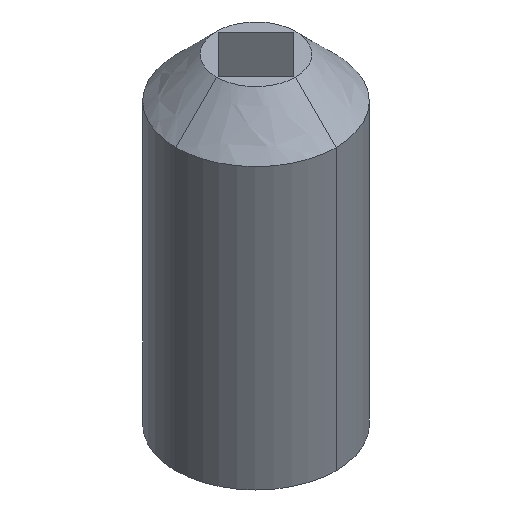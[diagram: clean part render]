
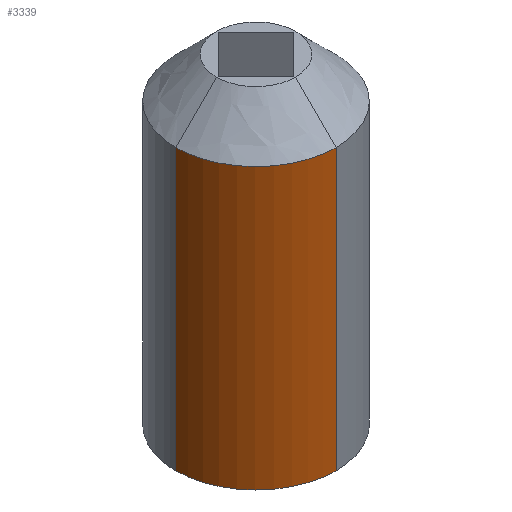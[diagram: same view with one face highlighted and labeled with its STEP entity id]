
A CAD part, isometric view. The second image highlights one B-rep face of the part: STEP entity #3339.
In plain terms, the highlighted free-form (B-spline) face has degree [2, 1] with [3, 2] control points.
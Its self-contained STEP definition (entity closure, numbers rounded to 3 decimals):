
#150 = VERTEX_POINT('',#151);
#151 = CARTESIAN_POINT('',(0.,-9.525,33.274));
#164 = ( BOUNDED_SURFACE() B_SPLINE_SURFACE(2,1,(
    (#165,#166)
    ,(#167,#168)
,(#169,#170
    )),.UNSPECIFIED.,.F.,.F.,.F.) B_SPLINE_SURFACE_WITH_KNOTS((3,3),(2,2
    ),(0.,1.),(0.,1.),.PIECEWISE_BEZIER_KNOTS.) 
GEOMETRIC_REPRESENTATION_ITEM() RATIONAL_B_SPLINE_SURFACE((
    (1.,1.)
    ,(0.707,0.707)
,(1.,1.))) REPRESENTATION_ITEM('') SURFACE() );
#165 = CARTESIAN_POINT('',(-4.699,0.,38.1));
#166 = CARTESIAN_POINT('',(-9.525,0.,33.274));
#167 = CARTESIAN_POINT('',(-4.699,-4.699,38.1));
#168 = CARTESIAN_POINT('',(-9.525,-9.525,33.274));
#169 = CARTESIAN_POINT('',(0.,-4.699,38.1));
#170 = CARTESIAN_POINT('',(0.,-9.525,33.274));
#214 = ( BOUNDED_SURFACE() B_SPLINE_SURFACE(2,1,(
    (#215,#216)
    ,(#217,#218)
,(#219,#220
    )),.UNSPECIFIED.,.F.,.F.,.F.) B_SPLINE_SURFACE_WITH_KNOTS((3,3),(2,2
    ),(0.,1.),(0.,1.),.PIECEWISE_BEZIER_KNOTS.) 
GEOMETRIC_REPRESENTATION_ITEM() RATIONAL_B_SPLINE_SURFACE((
    (1.,1.)
    ,(0.707,0.707)
,(1.,1.))) REPRESENTATION_ITEM('') SURFACE() );
#215 = CARTESIAN_POINT('',(0.,-9.525,33.274));
#216 = CARTESIAN_POINT('',(0.,-9.525,0.));
#217 = CARTESIAN_POINT('',(9.525,-9.525,33.274));
#218 = CARTESIAN_POINT('',(9.525,-9.525,0.));
#219 = CARTESIAN_POINT('',(9.525,0.,33.274));
#220 = CARTESIAN_POINT('',(9.525,0.,0.));
#1573 = VERTEX_POINT('',#1574);
#1574 = CARTESIAN_POINT('',(-9.525,0.,33.274));
#1608 = ( BOUNDED_SURFACE() B_SPLINE_SURFACE(2,1,(
    (#1609,#1610)
    ,(#1611,#1612)
    ,(#1613,#1614
)),.UNSPECIFIED.,.F.,.F.,.F.) B_SPLINE_SURFACE_WITH_KNOTS((3,3),(2,2),(
    0.,1.),(0.,1.),.PIECEWISE_BEZIER_KNOTS.) 
GEOMETRIC_REPRESENTATION_ITEM() RATIONAL_B_SPLINE_SURFACE((
    (1.,1.)
    ,(0.707,0.707)
,(1.,1.))) REPRESENTATION_ITEM('') SURFACE() );
#1609 = CARTESIAN_POINT('',(0.,9.525,33.274));
#1610 = CARTESIAN_POINT('',(0.,9.525,0.));
#1611 = CARTESIAN_POINT('',(-9.525,9.525,33.274));
#1612 = CARTESIAN_POINT('',(-9.525,9.525,0.));
#1613 = CARTESIAN_POINT('',(-9.525,0.,33.274));
#1614 = CARTESIAN_POINT('',(-9.525,0.,0.));
#1684 = PLANE('',#1685);
#1685 = AXIS2_PLACEMENT_3D('',#1686,#1687,#1688);
#1686 = CARTESIAN_POINT('',(9.525,0.,0.));
#1687 = DIRECTION('',(0.,0.,-1.));
#1688 = DIRECTION('',(-1.,0.,0.));
#1702 = EDGE_CURVE('',#1573,#150,#1703,.T.);
#1703 = SURFACE_CURVE('',#1704,(#1708,#1715),.PCURVE_S1.);
#1704 = ( BOUNDED_CURVE() B_SPLINE_CURVE(2,(#1705,#1706,#1707),
.UNSPECIFIED.,.F.,.F.) B_SPLINE_CURVE_WITH_KNOTS((3,3),(0.,1.),
.PIECEWISE_BEZIER_KNOTS.) CURVE() GEOMETRIC_REPRESENTATION_ITEM() 
RATIONAL_B_SPLINE_CURVE((1.,0.707,1.)) REPRESENTATION_ITEM('') 
  );
#1705 = CARTESIAN_POINT('',(-9.525,0.,33.274));
#1706 = CARTESIAN_POINT('',(-9.525,-9.525,33.274));
#1707 = CARTESIAN_POINT('',(0.,-9.525,33.274));
#1708 = PCURVE('',#164,#1709);
#1709 = DEFINITIONAL_REPRESENTATION('',(#1710),#1714);
#1710 = LINE('',#1711,#1712);
#1711 = CARTESIAN_POINT('',(0.,1.));
#1712 = VECTOR('',#1713,1.);
#1713 = DIRECTION('',(1.,0.));
#1714 = ( GEOMETRIC_REPRESENTATION_CONTEXT(2) 
PARAMETRIC_REPRESENTATION_CONTEXT() REPRESENTATION_CONTEXT('2D SPACE',''
  ) );
#1715 = PCURVE('',#1716,#1723);
#1716 = ( BOUNDED_SURFACE() B_SPLINE_SURFACE(2,1,(
    (#1717,#1718)
    ,(#1719,#1720)
    ,(#1721,#1722
)),.UNSPECIFIED.,.F.,.F.,.F.) B_SPLINE_SURFACE_WITH_KNOTS((3,3),(2,2),(
    0.,1.),(0.,1.),.PIECEWISE_BEZIER_KNOTS.) 
GEOMETRIC_REPRESENTATION_ITEM() RATIONAL_B_SPLINE_SURFACE((
    (1.,1.)
    ,(0.707,0.707)
,(1.,1.))) REPRESENTATION_ITEM('') SURFACE() );
#1717 = CARTESIAN_POINT('',(-9.525,0.,33.274));
#1718 = CARTESIAN_POINT('',(-9.525,0.,0.));
#1719 = CARTESIAN_POINT('',(-9.525,-9.525,33.274));
#1720 = CARTESIAN_POINT('',(-9.525,-9.525,0.));
#1721 = CARTESIAN_POINT('',(0.,-9.525,33.274));
#1722 = CARTESIAN_POINT('',(0.,-9.525,0.));
#1723 = DEFINITIONAL_REPRESENTATION('',(#1724),#1728);
#1724 = LINE('',#1725,#1726);
#1725 = CARTESIAN_POINT('',(0.,0.));
#1726 = VECTOR('',#1727,1.);
#1727 = DIRECTION('',(1.,0.));
#1728 = ( GEOMETRIC_REPRESENTATION_CONTEXT(2) 
PARAMETRIC_REPRESENTATION_CONTEXT() REPRESENTATION_CONTEXT('2D SPACE',''
  ) );
#1733 = EDGE_CURVE('',#150,#1734,#1736,.T.);
#1734 = VERTEX_POINT('',#1735);
#1735 = CARTESIAN_POINT('',(0.,-9.525,0.));
#1736 = SURFACE_CURVE('',#1737,(#1740,#1747),.PCURVE_S1.);
#1737 = B_SPLINE_CURVE_WITH_KNOTS('',1,(#1738,#1739),.UNSPECIFIED.,.F.,
  .F.,(2,2),(0.,1.),.PIECEWISE_BEZIER_KNOTS.);
#1738 = CARTESIAN_POINT('',(0.,-9.525,33.274));
#1739 = CARTESIAN_POINT('',(0.,-9.525,0.));
#1740 = PCURVE('',#214,#1741);
#1741 = DEFINITIONAL_REPRESENTATION('',(#1742),#1746);
#1742 = LINE('',#1743,#1744);
#1743 = CARTESIAN_POINT('',(0.,0.));
#1744 = VECTOR('',#1745,1.);
#1745 = DIRECTION('',(0.,1.));
#1746 = ( GEOMETRIC_REPRESENTATION_CONTEXT(2) 
PARAMETRIC_REPRESENTATION_CONTEXT() REPRESENTATION_CONTEXT('2D SPACE',''
  ) );
#1747 = PCURVE('',#1716,#1748);
#1748 = DEFINITIONAL_REPRESENTATION('',(#1749),#1753);
#1749 = LINE('',#1750,#1751);
#1750 = CARTESIAN_POINT('',(1.,0.));
#1751 = VECTOR('',#1752,1.);
#1752 = DIRECTION('',(0.,1.));
#1753 = ( GEOMETRIC_REPRESENTATION_CONTEXT(2) 
PARAMETRIC_REPRESENTATION_CONTEXT() REPRESENTATION_CONTEXT('2D SPACE',''
  ) );
#1972 = EDGE_CURVE('',#1573,#1973,#1975,.T.);
#1973 = VERTEX_POINT('',#1974);
#1974 = CARTESIAN_POINT('',(-9.525,0.,0.));
#1975 = SURFACE_CURVE('',#1976,(#1979,#1986),.PCURVE_S1.);
#1976 = B_SPLINE_CURVE_WITH_KNOTS('',1,(#1977,#1978),.UNSPECIFIED.,.F.,
  .F.,(2,2),(0.,1.),.PIECEWISE_BEZIER_KNOTS.);
#1977 = CARTESIAN_POINT('',(-9.525,0.,33.274));
#1978 = CARTESIAN_POINT('',(-9.525,0.,0.));
#1979 = PCURVE('',#1608,#1980);
#1980 = DEFINITIONAL_REPRESENTATION('',(#1981),#1985);
#1981 = LINE('',#1982,#1983);
#1982 = CARTESIAN_POINT('',(1.,0.));
#1983 = VECTOR('',#1984,1.);
#1984 = DIRECTION('',(0.,1.));
#1985 = ( GEOMETRIC_REPRESENTATION_CONTEXT(2) 
PARAMETRIC_REPRESENTATION_CONTEXT() REPRESENTATION_CONTEXT('2D SPACE',''
  ) );
#1986 = PCURVE('',#1716,#1987);
#1987 = DEFINITIONAL_REPRESENTATION('',(#1988),#1992);
#1988 = LINE('',#1989,#1990);
#1989 = CARTESIAN_POINT('',(0.,0.));
#1990 = VECTOR('',#1991,1.);
#1991 = DIRECTION('',(0.,1.));
#1992 = ( GEOMETRIC_REPRESENTATION_CONTEXT(2) 
PARAMETRIC_REPRESENTATION_CONTEXT() REPRESENTATION_CONTEXT('2D SPACE',''
  ) );
#3318 = EDGE_CURVE('',#1973,#1734,#3319,.T.);
#3319 = SURFACE_CURVE('',#3320,(#3324,#3331),.PCURVE_S1.);
#3320 = ( BOUNDED_CURVE() B_SPLINE_CURVE(2,(#3321,#3322,#3323),
.UNSPECIFIED.,.F.,.F.) B_SPLINE_CURVE_WITH_KNOTS((3,3),(0.,1.),
.PIECEWISE_BEZIER_KNOTS.) CURVE() GEOMETRIC_REPRESENTATION_ITEM() 
RATIONAL_B_SPLINE_CURVE((1.,0.707,1.)) REPRESENTATION_ITEM('') 
  );
#3321 = CARTESIAN_POINT('',(-9.525,0.,0.));
#3322 = CARTESIAN_POINT('',(-9.525,-9.525,0.));
#3323 = CARTESIAN_POINT('',(0.,-9.525,0.));
#3324 = PCURVE('',#1684,#3325);
#3325 = DEFINITIONAL_REPRESENTATION('',(#3326),#3330);
#3326 = ( BOUNDED_CURVE() B_SPLINE_CURVE(2,(#3327,#3328,#3329),
.UNSPECIFIED.,.F.,.F.) B_SPLINE_CURVE_WITH_KNOTS((3,3),(0.,1.),
.PIECEWISE_BEZIER_KNOTS.) CURVE() GEOMETRIC_REPRESENTATION_ITEM() 
RATIONAL_B_SPLINE_CURVE((1.,0.707,1.)) REPRESENTATION_ITEM('') 
  );
#3327 = CARTESIAN_POINT('',(19.05,0.));
#3328 = CARTESIAN_POINT('',(19.05,-9.525));
#3329 = CARTESIAN_POINT('',(9.525,-9.525));
#3330 = ( GEOMETRIC_REPRESENTATION_CONTEXT(2) 
PARAMETRIC_REPRESENTATION_CONTEXT() REPRESENTATION_CONTEXT('2D SPACE',''
  ) );
#3331 = PCURVE('',#1716,#3332);
#3332 = DEFINITIONAL_REPRESENTATION('',(#3333),#3337);
#3333 = LINE('',#3334,#3335);
#3334 = CARTESIAN_POINT('',(0.,1.));
#3335 = VECTOR('',#3336,1.);
#3336 = DIRECTION('',(1.,0.));
#3337 = ( GEOMETRIC_REPRESENTATION_CONTEXT(2) 
PARAMETRIC_REPRESENTATION_CONTEXT() REPRESENTATION_CONTEXT('2D SPACE',''
  ) );
#3339 = ADVANCED_FACE('',(#3340),#1716,.F.);
#3340 = FACE_BOUND('',#3341,.F.);
#3341 = EDGE_LOOP('',(#3342,#3343,#3344,#3345));
#3342 = ORIENTED_EDGE('',*,*,#1972,.F.);
#3343 = ORIENTED_EDGE('',*,*,#1702,.T.);
#3344 = ORIENTED_EDGE('',*,*,#1733,.T.);
#3345 = ORIENTED_EDGE('',*,*,#3318,.F.);
